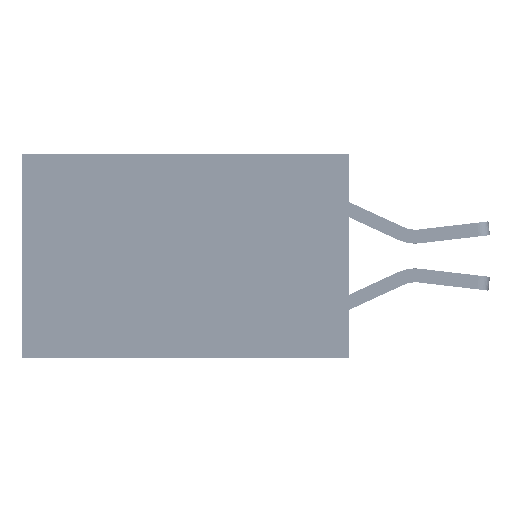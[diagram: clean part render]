
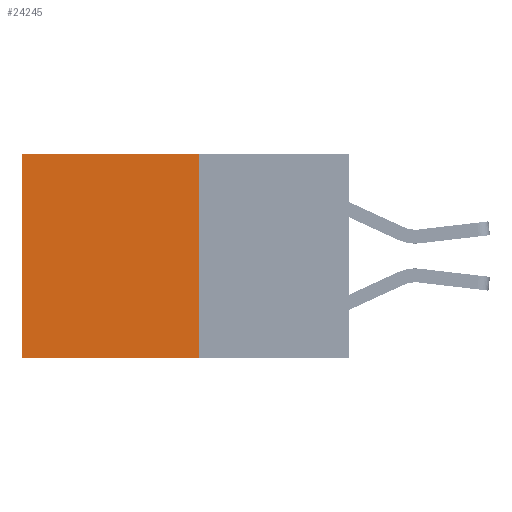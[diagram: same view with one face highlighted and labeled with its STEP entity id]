
A CAD part, left-side view. The second image highlights one B-rep face of the part: STEP entity #24245.
In plain terms, the highlighted planar face has unit normal (-1, 0, 0).
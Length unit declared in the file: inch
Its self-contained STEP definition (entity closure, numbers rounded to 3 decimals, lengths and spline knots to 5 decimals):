
#108 = DIRECTION ( 'NONE',  ( 1., 0., 0. ) ) ;
#427 = DIRECTION ( 'NONE',  ( 0., 1., 0. ) ) ;
#607 = LINE ( 'NONE', #15076, #13115 ) ;
#3472 = CARTESIAN_POINT ( 'NONE',  ( 0.277, 0.59, 0. ) ) ;
#4520 = CARTESIAN_POINT ( 'NONE',  ( 0.277, 0.59, -0.37 ) ) ;
#4980 = LINE ( 'NONE', #27204, #12908 ) ;
#5527 = VECTOR ( 'NONE', #20665, 39.37008 ) ;
#7222 = VERTEX_POINT ( 'NONE', #13237 ) ;
#7549 = ORIENTED_EDGE ( 'NONE', *, *, #15729, .F. ) ;
#7976 = CARTESIAN_POINT ( 'NONE',  ( 0.277, 0.59, -0.37 ) ) ;
#10101 = VERTEX_POINT ( 'NONE', #3472 ) ;
#10178 = ORIENTED_EDGE ( 'NONE', *, *, #26506, .T. ) ;
#12105 = EDGE_CURVE ( 'NONE', #7222, #10101, #4980, .T. ) ;
#12908 = VECTOR ( 'NONE', #427, 39.37008 ) ;
#13115 = VECTOR ( 'NONE', #33794, 39.37008 ) ;
#13237 = CARTESIAN_POINT ( 'NONE',  ( 0.277, 0.27, 0. ) ) ;
#15076 = CARTESIAN_POINT ( 'NONE',  ( 0.277, 0.27, -0.37 ) ) ;
#15729 = EDGE_CURVE ( 'NONE', #22632, #28693, #607, .T. ) ;
#15851 = ORIENTED_EDGE ( 'NONE', *, *, #12105, .T. ) ;
#16148 = CARTESIAN_POINT ( 'NONE',  ( 0.277, 0.27, -0.37 ) ) ;
#17790 = EDGE_LOOP ( 'NONE', ( #10178, #7549, #25356, #15851 ) ) ;
#18896 = DIRECTION ( 'NONE',  ( 0., 0., -1. ) ) ;
#20078 = EDGE_CURVE ( 'NONE', #7222, #22632, #29057, .T. ) ;
#20265 = VECTOR ( 'NONE', #34158, 39.37008 ) ;
#20665 = DIRECTION ( 'NONE',  ( 0., 0., -1. ) ) ;
#20680 = CARTESIAN_POINT ( 'NONE',  ( 0.277, 0.27, -0.37 ) ) ;
#20870 = FACE_OUTER_BOUND ( 'NONE', #17790, .T. ) ;
#22632 = VERTEX_POINT ( 'NONE', #20680 ) ;
#24245 = ADVANCED_FACE ( 'NONE', ( #20870 ), #26879, .F. ) ;
#25356 = ORIENTED_EDGE ( 'NONE', *, *, #20078, .F. ) ;
#25855 = AXIS2_PLACEMENT_3D ( 'NONE', #16148, #108, #18896 ) ;
#26506 = EDGE_CURVE ( 'NONE', #10101, #28693, #27813, .T. ) ;
#26879 = PLANE ( 'NONE',  #25855 ) ;
#27204 = CARTESIAN_POINT ( 'NONE',  ( 0.277, 0.27, 0. ) ) ;
#27813 = LINE ( 'NONE', #4520, #5527 ) ;
#28693 = VERTEX_POINT ( 'NONE', #7976 ) ;
#29057 = LINE ( 'NONE', #31529, #20265 ) ;
#31529 = CARTESIAN_POINT ( 'NONE',  ( 0.277, 0.27, -0.37 ) ) ;
#33794 = DIRECTION ( 'NONE',  ( 0., 1., 0. ) ) ;
#34158 = DIRECTION ( 'NONE',  ( 0., 0., -1. ) ) ;
